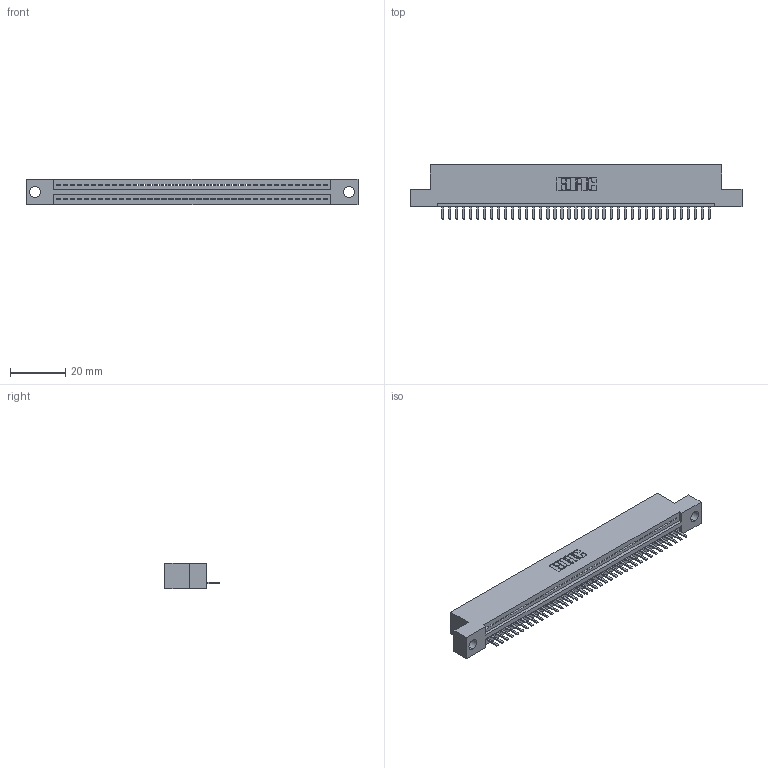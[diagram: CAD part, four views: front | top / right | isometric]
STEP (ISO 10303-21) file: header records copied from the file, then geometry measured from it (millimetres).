
FILE_DESCRIPTION (( 'STEP AP203' ), '1' );
FILE_NAME ('395-039-520-104.STEP', '2019-10-22T02:11:18', ( '' ), ( '' ), 'SwSTEP 2.0', 'SolidWorks 2016', '' );
FILE_SCHEMA (( 'CONFIG_CONTROL_DESIGN' ));
Length unit declared in the file: inch
Products named in the file (3): 345-292-001_345-293-120; 345 Part_Flush Mounting Lugs - 0.156 Dia-TH; 395-039-520-104
Assembly tree (40 placements, depth 2):
  395-039-520-104
    345 Part_Flush Mounting Lugs - 0.156 Dia-TH
    345-292-001_345-293-120  x39
Bounding box: 120.27 x 19.68 x 9.4 mm (x, y, z)
Volume: 11198.7 mm3; surface area: 14283 mm2
Topology: 40 solids, 40 shells, 2544 faces, 7517 edges, 4906 vertices
Faces by surface type: plane 1718, cylinder 826
Entity records: 29873 total; most frequent: CARTESIAN_POINT 5193, ORIENTED_EDGE 5154, DIRECTION 4527, EDGE_CURVE 2577, LINE 2285, VECTOR 2285, VERTEX_POINT 1714, AXIS2_PLACEMENT_3D 1121
